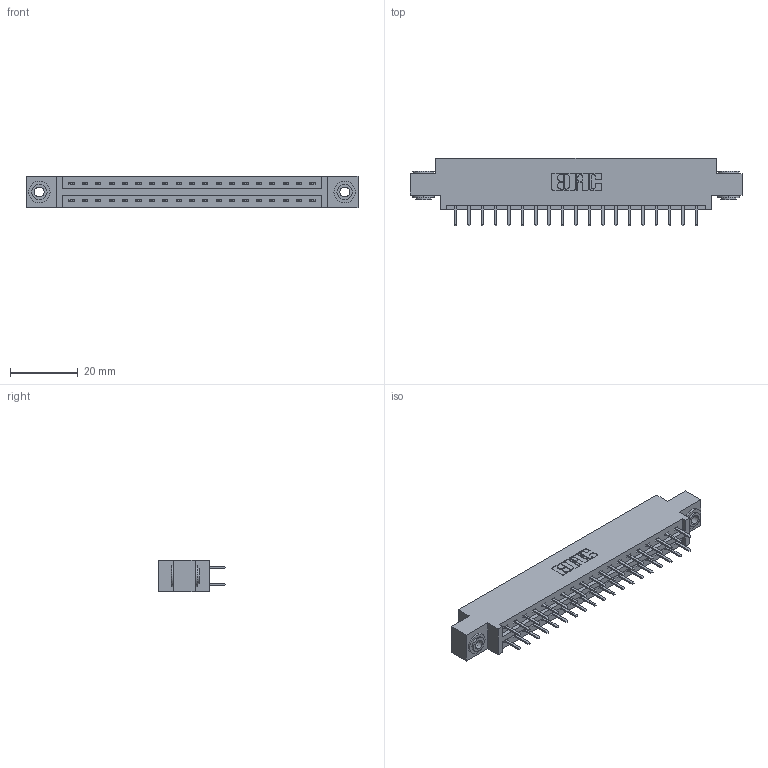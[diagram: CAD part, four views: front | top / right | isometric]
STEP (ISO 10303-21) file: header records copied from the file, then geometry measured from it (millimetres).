
FILE_DESCRIPTION (( 'STEP AP203' ), '1' );
FILE_NAME ('387-038-520-803.STEP', '2018-09-19T03:49:59', ( '' ), ( '' ), 'SwSTEP 2.0', 'SolidWorks 2016', '' );
FILE_SCHEMA (( 'CONFIG_CONTROL_DESIGN' ));
Length unit declared in the file: inch
Products named in the file (4): 337 Part_0.170 Offset - 0.156 Dia-TH; 345-292-001_345-293-120; 345-250-002_345-250-002-102; 387-038-520-803
Assembly tree (41 placements, depth 2):
  387-038-520-803
    337 Part_0.170 Offset - 0.156 Dia-TH
    345-292-001_345-293-120  x38
    345-250-002_345-250-002-102  x2
Bounding box: 98.3 x 20.02 x 9.4 mm (x, y, z)
Volume: 9938.5 mm3; surface area: 11296.6 mm2
Topology: 41 solids, 41 shells, 2360 faces, 6821 edges, 4442 vertices
Faces by surface type: plane 1604, cylinder 748, cone 8
Entity records: 18602 total; most frequent: CARTESIAN_POINT 3141, ORIENTED_EDGE 3058, DIRECTION 2735, EDGE_CURVE 1529, VECTOR 1373, LINE 1373, VERTEX_POINT 1014, AXIS2_PLACEMENT_3D 681
